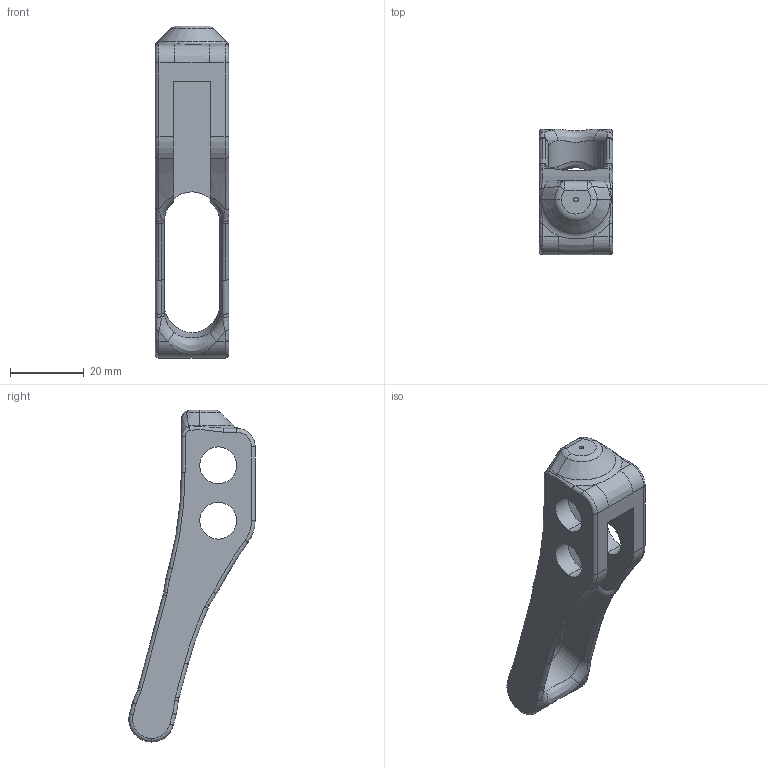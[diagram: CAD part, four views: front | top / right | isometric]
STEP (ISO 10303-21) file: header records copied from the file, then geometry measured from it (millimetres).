
FILE_DESCRIPTION (( 'STEP AP203' ), '1' );
FILE_NAME ('Hammer_Slide.STEP', '2013-11-14T05:06:45', ( '' ), ( '' ), 'SwSTEP 2.0', 'SolidWorks 2013', '' );
FILE_SCHEMA (( 'CONFIG_CONTROL_DESIGN' ));
Length unit declared in the file: millimetre
Products named in the file (1): Hammer_Slide
Bounding box: 19.9 x 34.22 x 90 mm (x, y, z)
Volume: 14199.6 mm3; surface area: 7573.4 mm2
Topology: 1 solids, 1 shells, 135 faces, 338 edges, 198 vertices
Faces by surface type: cylinder 42, bspline 38, torus 30, plane 20, cone 3, sphere 2
Entity records: 5245 total; most frequent: CARTESIAN_POINT 2119, ORIENTED_EDGE 672, DIRECTION 634, EDGE_CURVE 336, AXIS2_PLACEMENT_3D 275, VERTEX_POINT 198, CIRCLE 177, EDGE_LOOP 140
